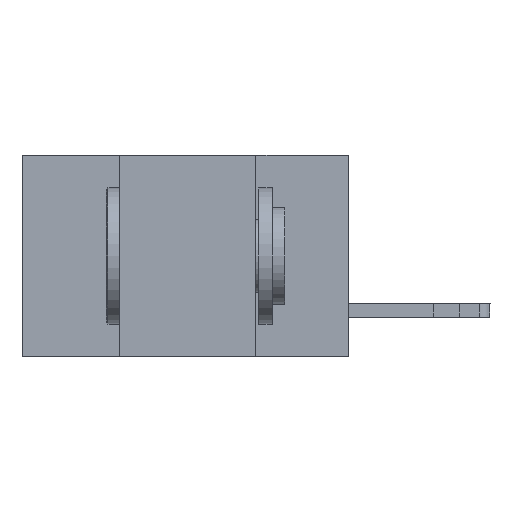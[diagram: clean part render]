
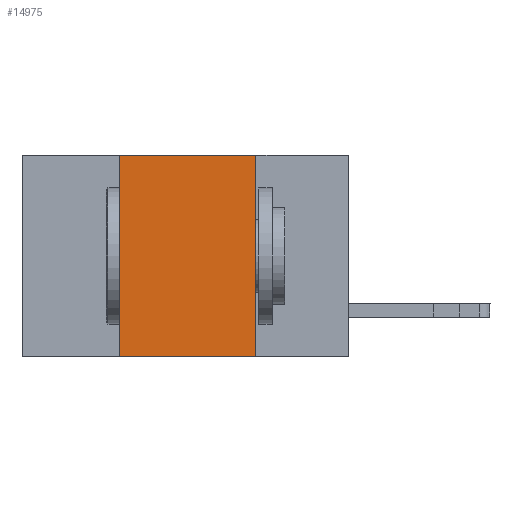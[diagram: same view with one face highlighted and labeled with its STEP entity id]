
A CAD part, left-side view. The second image highlights one B-rep face of the part: STEP entity #14975.
In plain terms, the highlighted planar face has unit normal (-1, 0, 0).
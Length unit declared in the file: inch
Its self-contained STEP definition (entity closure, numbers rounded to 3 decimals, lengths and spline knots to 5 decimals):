
#130 = DIRECTION ( 'NONE',  ( 0., 0., 1. ) ) ;
#832 = VECTOR ( 'NONE', #15716, 39.37008 ) ;
#1389 = VERTEX_POINT ( 'NONE', #8919 ) ;
#1498 = CARTESIAN_POINT ( 'NONE',  ( 0., 0.17, -0.37 ) ) ;
#1750 = CARTESIAN_POINT ( 'NONE',  ( 0., 0.6, -0.37 ) ) ;
#2249 = EDGE_CURVE ( 'NONE', #16663, #1389, #9042, .T. ) ;
#3008 = VECTOR ( 'NONE', #7386, 39.37008 ) ;
#3620 = VERTEX_POINT ( 'NONE', #5261 ) ;
#3646 = DIRECTION ( 'NONE',  ( 0., 0., -1. ) ) ;
#5261 = CARTESIAN_POINT ( 'NONE',  ( 0., 0.42, -0.37 ) ) ;
#5688 = VECTOR ( 'NONE', #9918, 39.37008 ) ;
#6114 = DIRECTION ( 'NONE',  ( 1., 0., 0. ) ) ;
#6578 = ORIENTED_EDGE ( 'NONE', *, *, #10758, .F. ) ;
#7386 = DIRECTION ( 'NONE',  ( 0., -1., 0. ) ) ;
#7493 = ORIENTED_EDGE ( 'NONE', *, *, #16998, .T. ) ;
#7808 = VECTOR ( 'NONE', #130, 39.37008 ) ;
#8237 = VERTEX_POINT ( 'NONE', #1498 ) ;
#8241 = LINE ( 'NONE', #11501, #7808 ) ;
#8919 = CARTESIAN_POINT ( 'NONE',  ( 0., 0.17, 0. ) ) ;
#8937 = CARTESIAN_POINT ( 'NONE',  ( 0., 0.6, 0. ) ) ;
#9042 = LINE ( 'NONE', #17234, #5688 ) ;
#9706 = ORIENTED_EDGE ( 'NONE', *, *, #10688, .F. ) ;
#9918 = DIRECTION ( 'NONE',  ( 0., -1., 0. ) ) ;
#10688 = EDGE_CURVE ( 'NONE', #3620, #16663, #8241, .T. ) ;
#10699 = AXIS2_PLACEMENT_3D ( 'NONE', #8937, #6114, #3646 ) ;
#10758 = EDGE_CURVE ( 'NONE', #1389, #8237, #17122, .T. ) ;
#10813 = PLANE ( 'NONE',  #10699 ) ;
#11501 = CARTESIAN_POINT ( 'NONE',  ( 0., 0.42, 0. ) ) ;
#13279 = CARTESIAN_POINT ( 'NONE',  ( 0., 0.42, 0. ) ) ;
#14284 = CARTESIAN_POINT ( 'NONE',  ( 0., 0.17, 0. ) ) ;
#14975 = ADVANCED_FACE ( 'NONE', ( #15197 ), #10813, .F. ) ;
#15197 = FACE_OUTER_BOUND ( 'NONE', #15540, .T. ) ;
#15540 = EDGE_LOOP ( 'NONE', ( #6578, #16217, #9706, #7493 ) ) ;
#15716 = DIRECTION ( 'NONE',  ( 0., 0., -1. ) ) ;
#16217 = ORIENTED_EDGE ( 'NONE', *, *, #2249, .F. ) ;
#16663 = VERTEX_POINT ( 'NONE', #13279 ) ;
#16998 = EDGE_CURVE ( 'NONE', #3620, #8237, #18135, .T. ) ;
#17122 = LINE ( 'NONE', #14284, #832 ) ;
#17234 = CARTESIAN_POINT ( 'NONE',  ( 0., 0.6, 0. ) ) ;
#18135 = LINE ( 'NONE', #1750, #3008 ) ;
